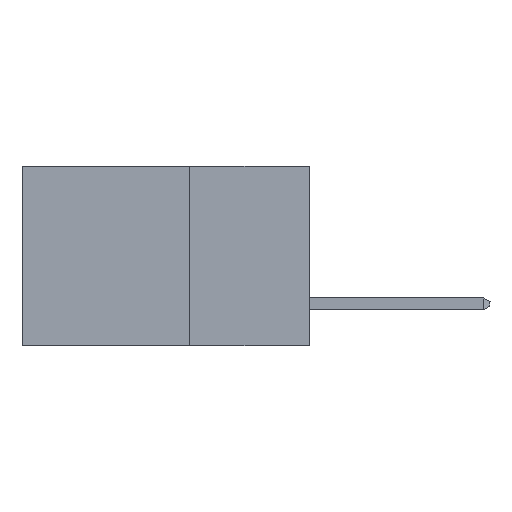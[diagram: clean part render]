
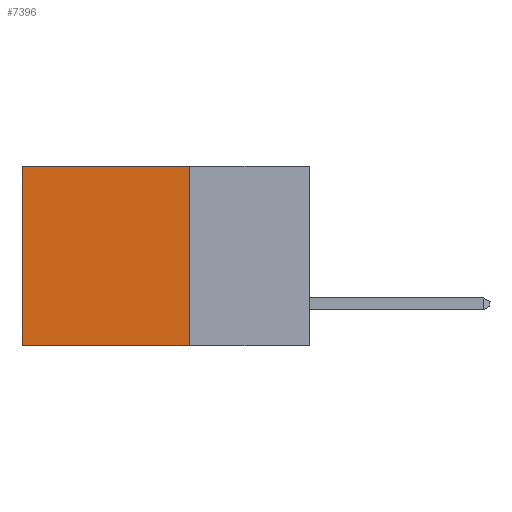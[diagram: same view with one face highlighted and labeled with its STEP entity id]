
A CAD part, left-side view. The second image highlights one B-rep face of the part: STEP entity #7396.
In plain terms, the highlighted planar face has unit normal (-1, 0, 0).
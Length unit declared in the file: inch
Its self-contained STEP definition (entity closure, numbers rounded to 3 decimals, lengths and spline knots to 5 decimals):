
#68 = CARTESIAN_POINT ( 'NONE',  ( 0.2875, 0.25, -0.375 ) ) ;
#334 = VECTOR ( 'NONE', #10522, 39.37008 ) ;
#643 = CARTESIAN_POINT ( 'NONE',  ( 0.2875, 0.25, -0.375 ) ) ;
#1271 = ORIENTED_EDGE ( 'NONE', *, *, #3656, .F. ) ;
#1620 = ORIENTED_EDGE ( 'NONE', *, *, #11266, .T. ) ;
#2841 = CARTESIAN_POINT ( 'NONE',  ( 0.2875, 0.25, 0. ) ) ;
#2868 = DIRECTION ( 'NONE',  ( 0., 0., -1. ) ) ;
#3021 = PLANE ( 'NONE',  #12499 ) ;
#3464 = LINE ( 'NONE', #9004, #12551 ) ;
#3656 = EDGE_CURVE ( 'NONE', #6719, #8194, #12207, .T. ) ;
#3785 = EDGE_LOOP ( 'NONE', ( #1620, #13488, #1271, #13635 ) ) ;
#4612 = DIRECTION ( 'NONE',  ( 0., 1., 0. ) ) ;
#4934 = CARTESIAN_POINT ( 'NONE',  ( 0.2875, 0.6, -0.375 ) ) ;
#5107 = LINE ( 'NONE', #15030, #334 ) ;
#5259 = FACE_OUTER_BOUND ( 'NONE', #3785, .T. ) ;
#5314 = CARTESIAN_POINT ( 'NONE',  ( 0.2875, 0.25, -0.375 ) ) ;
#6719 = VERTEX_POINT ( 'NONE', #2841 ) ;
#6767 = VECTOR ( 'NONE', #8494, 39.37008 ) ;
#6988 = EDGE_CURVE ( 'NONE', #8194, #11767, #3464, .T. ) ;
#7018 = EDGE_CURVE ( 'NONE', #6719, #14730, #5107, .T. ) ;
#7396 = ADVANCED_FACE ( 'NONE', ( #5259 ), #3021, .F. ) ;
#8194 = VERTEX_POINT ( 'NONE', #68 ) ;
#8494 = DIRECTION ( 'NONE',  ( 0., 0., -1. ) ) ;
#8677 = DIRECTION ( 'NONE',  ( 1., 0., 0. ) ) ;
#9004 = CARTESIAN_POINT ( 'NONE',  ( 0.2875, 0.25, -0.375 ) ) ;
#9848 = LINE ( 'NONE', #4934, #6767 ) ;
#10522 = DIRECTION ( 'NONE',  ( 0., 1., 0. ) ) ;
#10795 = CARTESIAN_POINT ( 'NONE',  ( 0.2875, 0.6, 0. ) ) ;
#11266 = EDGE_CURVE ( 'NONE', #14730, #11767, #9848, .T. ) ;
#11767 = VERTEX_POINT ( 'NONE', #11881 ) ;
#11881 = CARTESIAN_POINT ( 'NONE',  ( 0.2875, 0.6, -0.375 ) ) ;
#12207 = LINE ( 'NONE', #5314, #14570 ) ;
#12499 = AXIS2_PLACEMENT_3D ( 'NONE', #643, #8677, #2868 ) ;
#12551 = VECTOR ( 'NONE', #4612, 39.37008 ) ;
#13488 = ORIENTED_EDGE ( 'NONE', *, *, #6988, .F. ) ;
#13635 = ORIENTED_EDGE ( 'NONE', *, *, #7018, .T. ) ;
#14570 = VECTOR ( 'NONE', #14573, 39.37008 ) ;
#14573 = DIRECTION ( 'NONE',  ( 0., 0., -1. ) ) ;
#14730 = VERTEX_POINT ( 'NONE', #10795 ) ;
#15030 = CARTESIAN_POINT ( 'NONE',  ( 0.2875, 0.25, 0. ) ) ;
